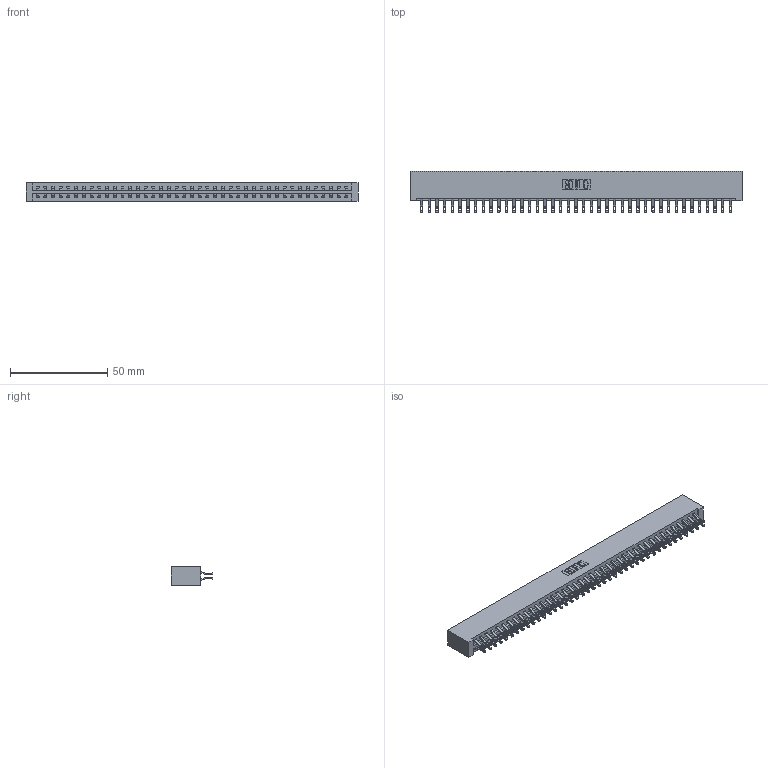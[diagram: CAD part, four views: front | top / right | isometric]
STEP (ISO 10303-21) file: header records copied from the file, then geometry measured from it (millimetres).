
FILE_DESCRIPTION (( 'STEP AP203' ), '1' );
FILE_NAME ('387-082-555-201.STEP', '2018-09-23T20:36:36', ( '' ), ( '' ), 'SwSTEP 2.0', 'SolidWorks 2016', '' );
FILE_SCHEMA (( 'CONFIG_CONTROL_DESIGN' ));
Length unit declared in the file: inch
Products named in the file (3): 337 Part_No Mounting Lugs; 345-292-001_555 Tail; 387-082-555-201
Assembly tree (83 placements, depth 2):
  387-082-555-201
    337 Part_No Mounting Lugs
    345-292-001_555 Tail  x82
Bounding box: 170.33 x 21.47 x 9.4 mm (x, y, z)
Volume: 18936.2 mm3; surface area: 22350.2 mm2
Topology: 83 solids, 83 shells, 5026 faces, 15785 edges, 10522 vertices
Faces by surface type: plane 3018, cylinder 2008
Entity records: 31967 total; most frequent: CARTESIAN_POINT 5420, ORIENTED_EDGE 5326, DIRECTION 4575, EDGE_CURVE 2663, LINE 2523, VECTOR 2523, VERTEX_POINT 1774, AXIS2_PLACEMENT_3D 1026
